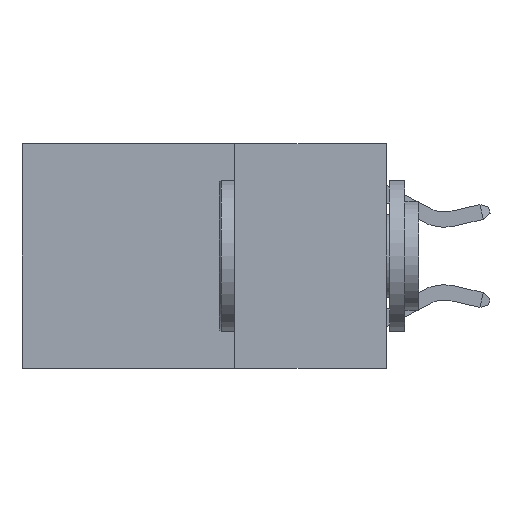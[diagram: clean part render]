
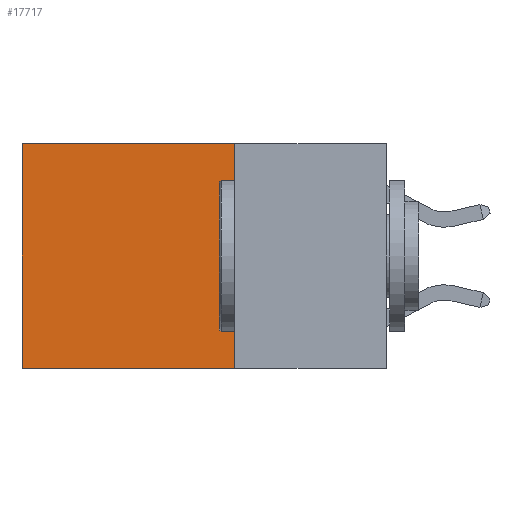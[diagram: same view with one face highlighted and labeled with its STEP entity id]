
A CAD part, left-side view. The second image highlights one B-rep face of the part: STEP entity #17717.
In plain terms, the highlighted planar face has unit normal (-1, 0, 0).
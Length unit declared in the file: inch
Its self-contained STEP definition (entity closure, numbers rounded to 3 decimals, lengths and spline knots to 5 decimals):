
#2044 = CARTESIAN_POINT ( 'NONE',  ( 0.2625, 0.25, 0. ) ) ;
#2232 = VECTOR ( 'NONE', #24577, 39.37008 ) ;
#2428 = CARTESIAN_POINT ( 'NONE',  ( 0.2625, 0.6, 0. ) ) ;
#2740 = LINE ( 'NONE', #11057, #7711 ) ;
#2805 = VECTOR ( 'NONE', #9285, 39.37008 ) ;
#5075 = ORIENTED_EDGE ( 'NONE', *, *, #13446, .T. ) ;
#5110 = VERTEX_POINT ( 'NONE', #14794 ) ;
#6871 = EDGE_CURVE ( 'NONE', #17914, #27485, #20883, .T. ) ;
#6889 = ORIENTED_EDGE ( 'NONE', *, *, #13710, .F. ) ;
#7039 = CARTESIAN_POINT ( 'NONE',  ( 0.2625, 0.6, 0. ) ) ;
#7711 = VECTOR ( 'NONE', #11419, 39.37008 ) ;
#9285 = DIRECTION ( 'NONE',  ( 0., 0., -1. ) ) ;
#10484 = EDGE_CURVE ( 'NONE', #5110, #27485, #13233, .T. ) ;
#11004 = CARTESIAN_POINT ( 'NONE',  ( 0.2625, 0.6, -0.37 ) ) ;
#11016 = VECTOR ( 'NONE', #20688, 39.37008 ) ;
#11057 = CARTESIAN_POINT ( 'NONE',  ( 0.2625, 0.25, 0. ) ) ;
#11419 = DIRECTION ( 'NONE',  ( 0., 1., 0. ) ) ;
#13233 = LINE ( 'NONE', #24675, #2232 ) ;
#13446 = EDGE_CURVE ( 'NONE', #22976, #17914, #2740, .T. ) ;
#13710 = EDGE_CURVE ( 'NONE', #22976, #5110, #22138, .T. ) ;
#14159 = CARTESIAN_POINT ( 'NONE',  ( 0.2625, 0.25, 0. ) ) ;
#14794 = CARTESIAN_POINT ( 'NONE',  ( 0.2625, 0.25, -0.37 ) ) ;
#15571 = EDGE_LOOP ( 'NONE', ( #15680, #17322, #6889, #5075 ) ) ;
#15680 = ORIENTED_EDGE ( 'NONE', *, *, #6871, .T. ) ;
#15964 = FACE_OUTER_BOUND ( 'NONE', #15571, .T. ) ;
#17322 = ORIENTED_EDGE ( 'NONE', *, *, #10484, .F. ) ;
#17717 = ADVANCED_FACE ( 'NONE', ( #15964 ), #19219, .F. ) ;
#17914 = VERTEX_POINT ( 'NONE', #2428 ) ;
#18263 = CARTESIAN_POINT ( 'NONE',  ( 0.2625, 0.25, 0. ) ) ;
#19219 = PLANE ( 'NONE',  #24655 ) ;
#20688 = DIRECTION ( 'NONE',  ( 0., 0., -1. ) ) ;
#20883 = LINE ( 'NONE', #7039, #2805 ) ;
#22138 = LINE ( 'NONE', #14159, #11016 ) ;
#22976 = VERTEX_POINT ( 'NONE', #18263 ) ;
#24577 = DIRECTION ( 'NONE',  ( 0., 1., 0. ) ) ;
#24655 = AXIS2_PLACEMENT_3D ( 'NONE', #2044, #27744, #25387 ) ;
#24675 = CARTESIAN_POINT ( 'NONE',  ( 0.2625, 0.25, -0.37 ) ) ;
#25387 = DIRECTION ( 'NONE',  ( 0., 0., -1. ) ) ;
#27485 = VERTEX_POINT ( 'NONE', #11004 ) ;
#27744 = DIRECTION ( 'NONE',  ( 1., 0., 0. ) ) ;
